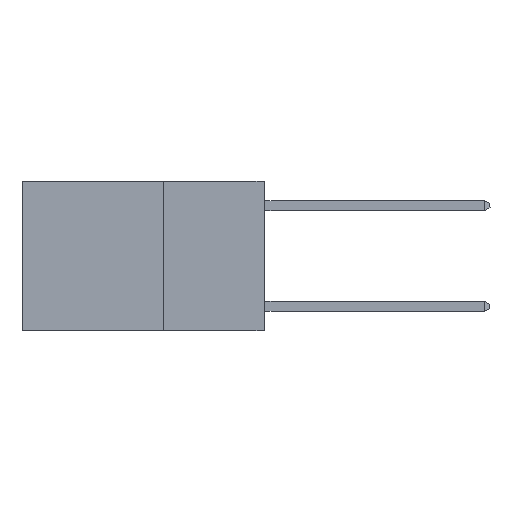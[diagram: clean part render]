
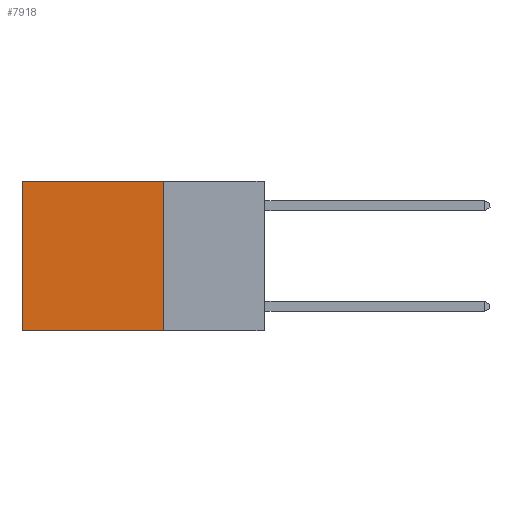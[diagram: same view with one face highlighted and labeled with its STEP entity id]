
A CAD part, left-side view. The second image highlights one B-rep face of the part: STEP entity #7918.
In plain terms, the highlighted planar face has unit normal (-1, 0, 0).
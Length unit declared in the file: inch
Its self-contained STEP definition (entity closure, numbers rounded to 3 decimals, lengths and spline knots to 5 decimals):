
#240 = AXIS2_PLACEMENT_3D ( 'NONE', #1298, #5309, #8133 ) ;
#377 = VERTEX_POINT ( 'NONE', #4872 ) ;
#501 = ORIENTED_EDGE ( 'NONE', *, *, #5436, .F. ) ;
#595 = VECTOR ( 'NONE', #6796, 39.37008 ) ;
#643 = CARTESIAN_POINT ( 'NONE',  ( 0.2625, 0.25, 0. ) ) ;
#1028 = LINE ( 'NONE', #10225, #595 ) ;
#1215 = EDGE_CURVE ( 'NONE', #8976, #4873, #1028, .T. ) ;
#1298 = CARTESIAN_POINT ( 'NONE',  ( 0.2625, 0.25, 0. ) ) ;
#1562 = EDGE_LOOP ( 'NONE', ( #9205, #12134, #501, #7379 ) ) ;
#3885 = LINE ( 'NONE', #4205, #10644 ) ;
#4062 = CARTESIAN_POINT ( 'NONE',  ( 0.2625, 0.25, -0.37 ) ) ;
#4205 = CARTESIAN_POINT ( 'NONE',  ( 0.2625, 0.25, 0. ) ) ;
#4449 = LINE ( 'NONE', #9870, #5468 ) ;
#4872 = CARTESIAN_POINT ( 'NONE',  ( 0.2625, 0.6, -0.37 ) ) ;
#4873 = VERTEX_POINT ( 'NONE', #11957 ) ;
#5309 = DIRECTION ( 'NONE',  ( 1., 0., 0. ) ) ;
#5436 = EDGE_CURVE ( 'NONE', #8976, #12320, #3885, .T. ) ;
#5468 = VECTOR ( 'NONE', #10688, 39.37008 ) ;
#6034 = PLANE ( 'NONE',  #240 ) ;
#6096 = DIRECTION ( 'NONE',  ( 0., 0., -1. ) ) ;
#6527 = FACE_OUTER_BOUND ( 'NONE', #1562, .T. ) ;
#6796 = DIRECTION ( 'NONE',  ( 0., 1., 0. ) ) ;
#7379 = ORIENTED_EDGE ( 'NONE', *, *, #1215, .T. ) ;
#7445 = CARTESIAN_POINT ( 'NONE',  ( 0.2625, 0.25, -0.37 ) ) ;
#7918 = ADVANCED_FACE ( 'NONE', ( #6527 ), #6034, .F. ) ;
#8133 = DIRECTION ( 'NONE',  ( 0., 0., -1. ) ) ;
#8922 = LINE ( 'NONE', #7445, #9376 ) ;
#8976 = VERTEX_POINT ( 'NONE', #643 ) ;
#9205 = ORIENTED_EDGE ( 'NONE', *, *, #12343, .T. ) ;
#9376 = VECTOR ( 'NONE', #12114, 39.37008 ) ;
#9870 = CARTESIAN_POINT ( 'NONE',  ( 0.2625, 0.6, 0. ) ) ;
#10225 = CARTESIAN_POINT ( 'NONE',  ( 0.2625, 0.25, 0. ) ) ;
#10644 = VECTOR ( 'NONE', #6096, 39.37008 ) ;
#10688 = DIRECTION ( 'NONE',  ( 0., 0., -1. ) ) ;
#11258 = EDGE_CURVE ( 'NONE', #12320, #377, #8922, .T. ) ;
#11957 = CARTESIAN_POINT ( 'NONE',  ( 0.2625, 0.6, 0. ) ) ;
#12114 = DIRECTION ( 'NONE',  ( 0., 1., 0. ) ) ;
#12134 = ORIENTED_EDGE ( 'NONE', *, *, #11258, .F. ) ;
#12320 = VERTEX_POINT ( 'NONE', #4062 ) ;
#12343 = EDGE_CURVE ( 'NONE', #4873, #377, #4449, .T. ) ;
